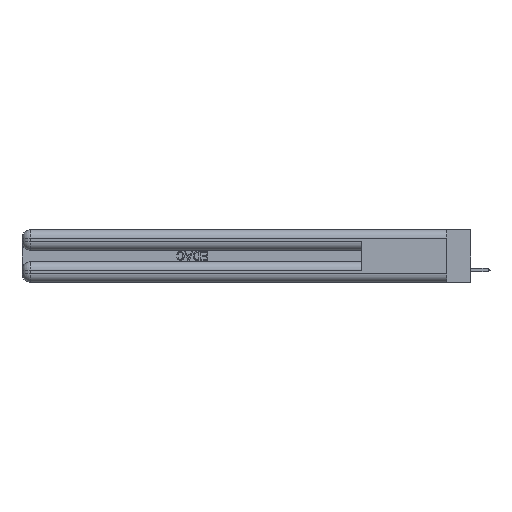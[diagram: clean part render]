
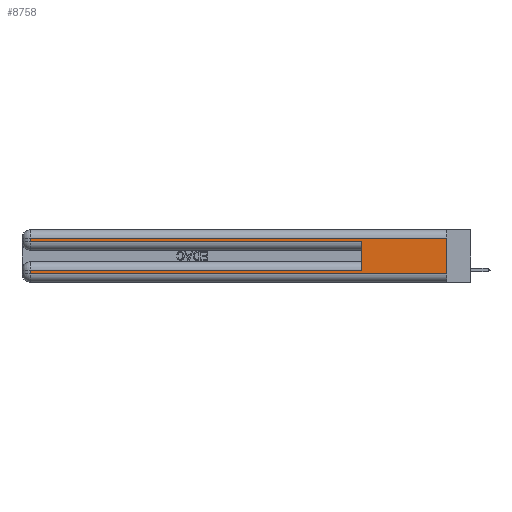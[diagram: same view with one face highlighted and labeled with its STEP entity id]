
A CAD part, left-side view. The second image highlights one B-rep face of the part: STEP entity #8758.
In plain terms, the highlighted planar face has unit normal (-1, 0, 0).
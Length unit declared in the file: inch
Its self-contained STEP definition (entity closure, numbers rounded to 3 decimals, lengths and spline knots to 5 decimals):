
#16 = LINE ( 'NONE', #17728, #37767 ) ;
#136 = VERTEX_POINT ( 'NONE', #21556 ) ;
#348 = DIRECTION ( 'NONE',  ( 0., 0., -1. ) ) ;
#1033 = ORIENTED_EDGE ( 'NONE', *, *, #25788, .T. ) ;
#1644 = VECTOR ( 'NONE', #20203, 39.37008 ) ;
#1868 = DIRECTION ( 'NONE',  ( 0., 0., 1. ) ) ;
#2137 = CARTESIAN_POINT ( 'NONE',  ( 0., 0.6, 0.145 ) ) ;
#2317 = CARTESIAN_POINT ( 'NONE',  ( 0., 0., 0.06 ) ) ;
#2777 = CARTESIAN_POINT ( 'NONE',  ( 0., 2.94, 0.085 ) ) ;
#2845 = DIRECTION ( 'NONE',  ( 0., -1., 0. ) ) ;
#2970 = LINE ( 'NONE', #2137, #39270 ) ;
#3429 = CARTESIAN_POINT ( 'NONE',  ( 0., 0., 0.085 ) ) ;
#4116 = CARTESIAN_POINT ( 'NONE',  ( 0., 0., 0.285 ) ) ;
#4556 = DIRECTION ( 'NONE',  ( 0., 0., -1. ) ) ;
#4679 = CARTESIAN_POINT ( 'NONE',  ( 0., 2.94, 0.37 ) ) ;
#5585 = ORIENTED_EDGE ( 'NONE', *, *, #6127, .T. ) ;
#6127 = EDGE_CURVE ( 'NONE', #18791, #36237, #23692, .T. ) ;
#7386 = DIRECTION ( 'NONE',  ( 1., 0., 0. ) ) ;
#8131 = EDGE_CURVE ( 'NONE', #28344, #38122, #28865, .T. ) ;
#8758 = ADVANCED_FACE ( 'NONE', ( #37668 ), #22843, .F. ) ;
#9478 = LINE ( 'NONE', #22957, #1644 ) ;
#12710 = VECTOR ( 'NONE', #38910, 39.37008 ) ;
#13516 = EDGE_CURVE ( 'NONE', #136, #28344, #9478, .T. ) ;
#14775 = CARTESIAN_POINT ( 'NONE',  ( 0., 2.94, 0.06 ) ) ;
#15784 = VECTOR ( 'NONE', #35607, 39.37008 ) ;
#17728 = CARTESIAN_POINT ( 'NONE',  ( 0., 0., 0.37 ) ) ;
#18479 = AXIS2_PLACEMENT_3D ( 'NONE', #38685, #7386, #348 ) ;
#18791 = VERTEX_POINT ( 'NONE', #32617 ) ;
#19957 = ORIENTED_EDGE ( 'NONE', *, *, #30624, .T. ) ;
#20041 = VERTEX_POINT ( 'NONE', #14775 ) ;
#20109 = ORIENTED_EDGE ( 'NONE', *, *, #39829, .T. ) ;
#20203 = DIRECTION ( 'NONE',  ( 0., 0., -1. ) ) ;
#20350 = ORIENTED_EDGE ( 'NONE', *, *, #20695, .F. ) ;
#20695 = EDGE_CURVE ( 'NONE', #39968, #27880, #16, .T. ) ;
#21556 = CARTESIAN_POINT ( 'NONE',  ( 0., 2.94, 0.31 ) ) ;
#22672 = VECTOR ( 'NONE', #26134, 39.37008 ) ;
#22843 = PLANE ( 'NONE',  #18479 ) ;
#22957 = CARTESIAN_POINT ( 'NONE',  ( 0., 2.94, 0.37 ) ) ;
#23692 = LINE ( 'NONE', #3429, #22672 ) ;
#24112 = LINE ( 'NONE', #38505, #15784 ) ;
#25788 = EDGE_CURVE ( 'NONE', #39968, #136, #24112, .T. ) ;
#26134 = DIRECTION ( 'NONE',  ( 0., 1., 0. ) ) ;
#27880 = VERTEX_POINT ( 'NONE', #2317 ) ;
#27974 = EDGE_LOOP ( 'NONE', ( #20350, #1033, #32080, #39580, #39422, #5585, #19957, #20109 ) ) ;
#28344 = VERTEX_POINT ( 'NONE', #32118 ) ;
#28865 = LINE ( 'NONE', #4116, #12710 ) ;
#29007 = LINE ( 'NONE', #34211, #30482 ) ;
#30482 = VECTOR ( 'NONE', #2845, 39.37008 ) ;
#30624 = EDGE_CURVE ( 'NONE', #36237, #20041, #40423, .T. ) ;
#32080 = ORIENTED_EDGE ( 'NONE', *, *, #13516, .T. ) ;
#32118 = CARTESIAN_POINT ( 'NONE',  ( 0., 2.94, 0.285 ) ) ;
#32617 = CARTESIAN_POINT ( 'NONE',  ( 0., 0.6, 0.085 ) ) ;
#34211 = CARTESIAN_POINT ( 'NONE',  ( 0., 0., 0.06 ) ) ;
#35111 = CARTESIAN_POINT ( 'NONE',  ( 0., 0.6, 0.285 ) ) ;
#35517 = EDGE_CURVE ( 'NONE', #18791, #38122, #2970, .T. ) ;
#35607 = DIRECTION ( 'NONE',  ( 0., 1., 0. ) ) ;
#36237 = VERTEX_POINT ( 'NONE', #2777 ) ;
#36978 = VECTOR ( 'NONE', #4556, 39.37008 ) ;
#37668 = FACE_OUTER_BOUND ( 'NONE', #27974, .T. ) ;
#37767 = VECTOR ( 'NONE', #39707, 39.37008 ) ;
#38122 = VERTEX_POINT ( 'NONE', #35111 ) ;
#38162 = CARTESIAN_POINT ( 'NONE',  ( 0., 0., 0.31 ) ) ;
#38505 = CARTESIAN_POINT ( 'NONE',  ( 0., 0., 0.31 ) ) ;
#38685 = CARTESIAN_POINT ( 'NONE',  ( 0., 0., 0.37 ) ) ;
#38910 = DIRECTION ( 'NONE',  ( 0., -1., 0. ) ) ;
#39270 = VECTOR ( 'NONE', #1868, 39.37008 ) ;
#39422 = ORIENTED_EDGE ( 'NONE', *, *, #35517, .F. ) ;
#39580 = ORIENTED_EDGE ( 'NONE', *, *, #8131, .T. ) ;
#39707 = DIRECTION ( 'NONE',  ( 0., 0., -1. ) ) ;
#39829 = EDGE_CURVE ( 'NONE', #20041, #27880, #29007, .T. ) ;
#39968 = VERTEX_POINT ( 'NONE', #38162 ) ;
#40423 = LINE ( 'NONE', #4679, #36978 ) ;
